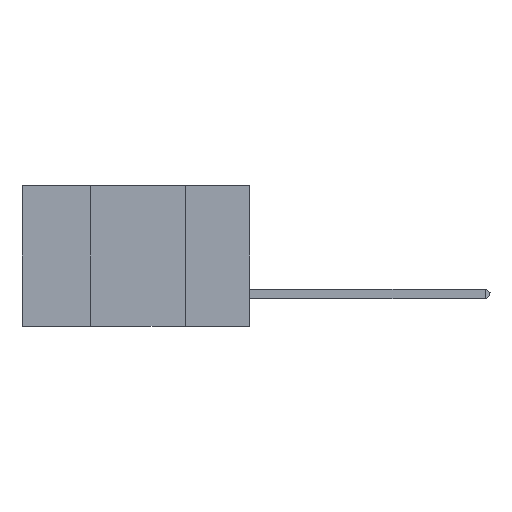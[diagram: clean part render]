
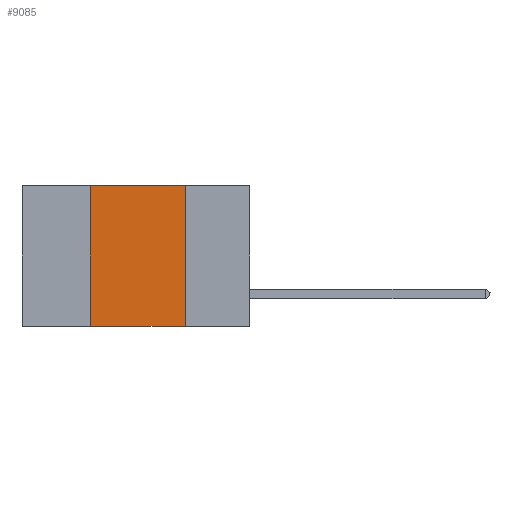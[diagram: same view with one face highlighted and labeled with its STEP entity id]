
A CAD part, left-side view. The second image highlights one B-rep face of the part: STEP entity #9085.
In plain terms, the highlighted planar face has unit normal (-1, 0, 0).
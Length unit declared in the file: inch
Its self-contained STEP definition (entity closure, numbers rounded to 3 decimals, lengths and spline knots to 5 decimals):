
#599 = LINE ( 'NONE', #1619, #7018 ) ;
#1023 = VERTEX_POINT ( 'NONE', #3006 ) ;
#1366 = VECTOR ( 'NONE', #4197, 39.37008 ) ;
#1619 = CARTESIAN_POINT ( 'NONE',  ( 0., 0.6, -0.37 ) ) ;
#2774 = CARTESIAN_POINT ( 'NONE',  ( 0., 0.17, 0. ) ) ;
#2876 = EDGE_LOOP ( 'NONE', ( #4403, #3910, #11765, #3277 ) ) ;
#3006 = CARTESIAN_POINT ( 'NONE',  ( 0., 0.17, 0. ) ) ;
#3277 = ORIENTED_EDGE ( 'NONE', *, *, #6402, .T. ) ;
#3296 = DIRECTION ( 'NONE',  ( 1., 0., 0. ) ) ;
#3471 = PLANE ( 'NONE',  #5508 ) ;
#3910 = ORIENTED_EDGE ( 'NONE', *, *, #11729, .F. ) ;
#4073 = LINE ( 'NONE', #7943, #5159 ) ;
#4131 = LINE ( 'NONE', #7766, #1366 ) ;
#4197 = DIRECTION ( 'NONE',  ( 0., 0., 1. ) ) ;
#4199 = FACE_OUTER_BOUND ( 'NONE', #2876, .T. ) ;
#4267 = VERTEX_POINT ( 'NONE', #6931 ) ;
#4403 = ORIENTED_EDGE ( 'NONE', *, *, #5813, .F. ) ;
#4525 = VECTOR ( 'NONE', #6390, 39.37008 ) ;
#5159 = VECTOR ( 'NONE', #11533, 39.37008 ) ;
#5258 = DIRECTION ( 'NONE',  ( 0., 0., -1. ) ) ;
#5504 = LINE ( 'NONE', #2774, #4525 ) ;
#5508 = AXIS2_PLACEMENT_3D ( 'NONE', #6151, #3296, #5258 ) ;
#5813 = EDGE_CURVE ( 'NONE', #1023, #9673, #5504, .T. ) ;
#6061 = VERTEX_POINT ( 'NONE', #10615 ) ;
#6151 = CARTESIAN_POINT ( 'NONE',  ( 0., 0.6, 0. ) ) ;
#6237 = CARTESIAN_POINT ( 'NONE',  ( 0., 0.17, -0.37 ) ) ;
#6390 = DIRECTION ( 'NONE',  ( 0., 0., -1. ) ) ;
#6402 = EDGE_CURVE ( 'NONE', #4267, #9673, #599, .T. ) ;
#6931 = CARTESIAN_POINT ( 'NONE',  ( 0., 0.42, -0.37 ) ) ;
#7018 = VECTOR ( 'NONE', #7810, 39.37008 ) ;
#7766 = CARTESIAN_POINT ( 'NONE',  ( 0., 0.42, 0. ) ) ;
#7810 = DIRECTION ( 'NONE',  ( 0., -1., 0. ) ) ;
#7943 = CARTESIAN_POINT ( 'NONE',  ( 0., 0.6, 0. ) ) ;
#9085 = ADVANCED_FACE ( 'NONE', ( #4199 ), #3471, .F. ) ;
#9673 = VERTEX_POINT ( 'NONE', #6237 ) ;
#10615 = CARTESIAN_POINT ( 'NONE',  ( 0., 0.42, 0. ) ) ;
#11533 = DIRECTION ( 'NONE',  ( 0., -1., 0. ) ) ;
#11729 = EDGE_CURVE ( 'NONE', #6061, #1023, #4073, .T. ) ;
#11765 = ORIENTED_EDGE ( 'NONE', *, *, #11787, .F. ) ;
#11787 = EDGE_CURVE ( 'NONE', #4267, #6061, #4131, .T. ) ;
